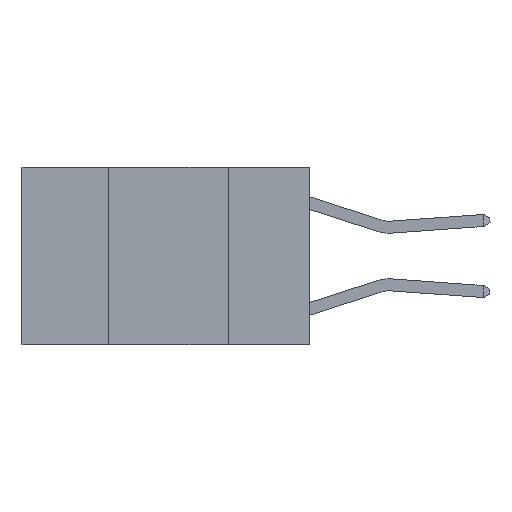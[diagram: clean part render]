
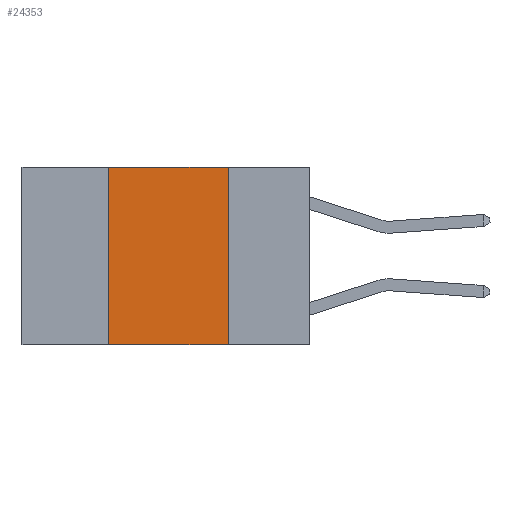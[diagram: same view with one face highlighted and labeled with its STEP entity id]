
A CAD part, left-side view. The second image highlights one B-rep face of the part: STEP entity #24353.
In plain terms, the highlighted planar face has unit normal (-1, 0, 0).
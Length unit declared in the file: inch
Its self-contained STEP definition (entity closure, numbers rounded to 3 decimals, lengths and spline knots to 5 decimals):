
#1867 = EDGE_CURVE ( 'NONE', #22327, #6350, #19435, .T. ) ;
#3723 = VECTOR ( 'NONE', #22538, 39.37008 ) ;
#3972 = CARTESIAN_POINT ( 'NONE',  ( 0., 0.42, -0.37 ) ) ;
#4730 = ORIENTED_EDGE ( 'NONE', *, *, #4752, .F. ) ;
#4752 = EDGE_CURVE ( 'NONE', #16478, #25390, #27217, .T. ) ;
#5848 = CARTESIAN_POINT ( 'NONE',  ( 0., 0.17, -0.37 ) ) ;
#6155 = CARTESIAN_POINT ( 'NONE',  ( 0., 0.42, 0. ) ) ;
#6350 = VERTEX_POINT ( 'NONE', #5848 ) ;
#6438 = EDGE_LOOP ( 'NONE', ( #15579, #17117, #4730, #10182 ) ) ;
#7764 = EDGE_CURVE ( 'NONE', #25390, #22327, #24496, .T. ) ;
#8007 = VECTOR ( 'NONE', #22435, 39.37008 ) ;
#8182 = EDGE_CURVE ( 'NONE', #16478, #6350, #16505, .T. ) ;
#9875 = CARTESIAN_POINT ( 'NONE',  ( 0., 0.42, 0. ) ) ;
#10182 = ORIENTED_EDGE ( 'NONE', *, *, #8182, .T. ) ;
#10750 = DIRECTION ( 'NONE',  ( 1., 0., 0. ) ) ;
#14208 = DIRECTION ( 'NONE',  ( 0., 0., 1. ) ) ;
#15579 = ORIENTED_EDGE ( 'NONE', *, *, #1867, .F. ) ;
#16442 = FACE_OUTER_BOUND ( 'NONE', #6438, .T. ) ;
#16478 = VERTEX_POINT ( 'NONE', #3972 ) ;
#16505 = LINE ( 'NONE', #20410, #3723 ) ;
#17004 = CARTESIAN_POINT ( 'NONE',  ( 0., 0.6, 0. ) ) ;
#17117 = ORIENTED_EDGE ( 'NONE', *, *, #7764, .F. ) ;
#17123 = CARTESIAN_POINT ( 'NONE',  ( 0., 0.6, 0. ) ) ;
#18186 = CARTESIAN_POINT ( 'NONE',  ( 0., 0.17, 0. ) ) ;
#18809 = CARTESIAN_POINT ( 'NONE',  ( 0., 0.17, 0. ) ) ;
#18885 = VECTOR ( 'NONE', #25578, 39.37008 ) ;
#19435 = LINE ( 'NONE', #18186, #8007 ) ;
#20410 = CARTESIAN_POINT ( 'NONE',  ( 0., 0.6, -0.37 ) ) ;
#20687 = AXIS2_PLACEMENT_3D ( 'NONE', #17123, #10750, #25609 ) ;
#22327 = VERTEX_POINT ( 'NONE', #18809 ) ;
#22435 = DIRECTION ( 'NONE',  ( 0., 0., -1. ) ) ;
#22538 = DIRECTION ( 'NONE',  ( 0., -1., 0. ) ) ;
#23509 = PLANE ( 'NONE',  #20687 ) ;
#24353 = ADVANCED_FACE ( 'NONE', ( #16442 ), #23509, .F. ) ;
#24496 = LINE ( 'NONE', #17004, #18885 ) ;
#25390 = VERTEX_POINT ( 'NONE', #6155 ) ;
#25578 = DIRECTION ( 'NONE',  ( 0., -1., 0. ) ) ;
#25609 = DIRECTION ( 'NONE',  ( 0., 0., -1. ) ) ;
#26584 = VECTOR ( 'NONE', #14208, 39.37008 ) ;
#27217 = LINE ( 'NONE', #9875, #26584 ) ;
